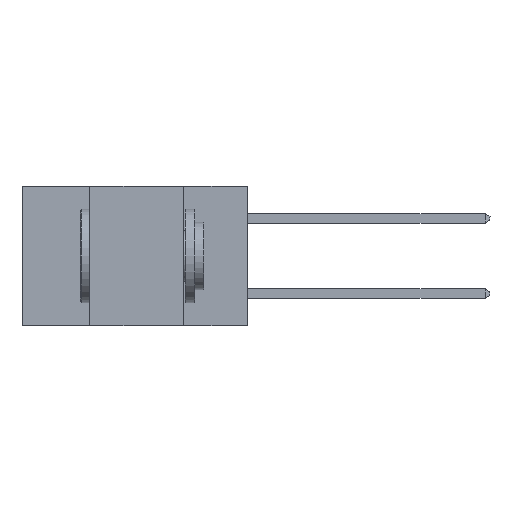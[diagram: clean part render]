
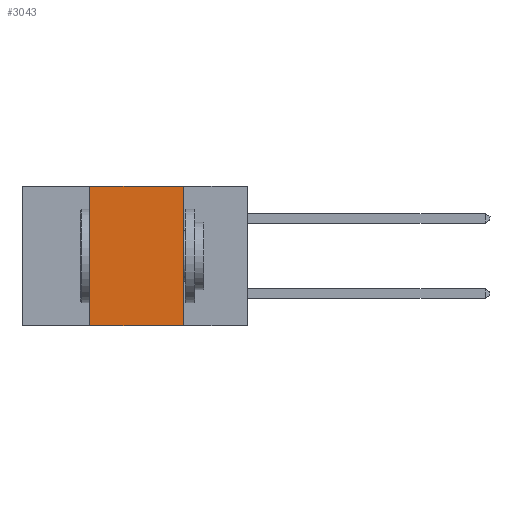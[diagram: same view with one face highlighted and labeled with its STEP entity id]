
A CAD part, left-side view. The second image highlights one B-rep face of the part: STEP entity #3043.
In plain terms, the highlighted planar face has unit normal (-1, 0, 0).
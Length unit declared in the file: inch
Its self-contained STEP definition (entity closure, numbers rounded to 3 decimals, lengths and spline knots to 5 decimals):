
#281 = EDGE_CURVE ( 'NONE', #7087, #9603, #7004, .T. ) ;
#705 = LINE ( 'NONE', #3749, #7884 ) ;
#1080 = PLANE ( 'NONE',  #6649 ) ;
#1147 = EDGE_CURVE ( 'NONE', #7087, #3100, #9301, .T. ) ;
#1456 = VERTEX_POINT ( 'NONE', #3692 ) ;
#1978 = DIRECTION ( 'NONE',  ( 1., 0., 0. ) ) ;
#2467 = DIRECTION ( 'NONE',  ( 0., 0., 1. ) ) ;
#2576 = FACE_OUTER_BOUND ( 'NONE', #8506, .T. ) ;
#3043 = ADVANCED_FACE ( 'NONE', ( #2576 ), #1080, .F. ) ;
#3100 = VERTEX_POINT ( 'NONE', #5658 ) ;
#3257 = LINE ( 'NONE', #4145, #5069 ) ;
#3325 = CARTESIAN_POINT ( 'NONE',  ( 0., 0.42, -0.37 ) ) ;
#3459 = ORIENTED_EDGE ( 'NONE', *, *, #281, .T. ) ;
#3510 = EDGE_CURVE ( 'NONE', #1456, #9603, #3257, .T. ) ;
#3692 = CARTESIAN_POINT ( 'NONE',  ( 0., 0.17, 0. ) ) ;
#3749 = CARTESIAN_POINT ( 'NONE',  ( 0., 0.6, 0. ) ) ;
#4145 = CARTESIAN_POINT ( 'NONE',  ( 0., 0.17, -0.37 ) ) ;
#4190 = DIRECTION ( 'NONE',  ( 0., 0., -1. ) ) ;
#4514 = CARTESIAN_POINT ( 'NONE',  ( 0., 0.17, -0.37 ) ) ;
#5069 = VECTOR ( 'NONE', #4190, 39.37008 ) ;
#5538 = ORIENTED_EDGE ( 'NONE', *, *, #7918, .F. ) ;
#5658 = CARTESIAN_POINT ( 'NONE',  ( 0., 0.42, 0. ) ) ;
#6241 = ORIENTED_EDGE ( 'NONE', *, *, #1147, .F. ) ;
#6649 = AXIS2_PLACEMENT_3D ( 'NONE', #8657, #1978, #8007 ) ;
#7004 = LINE ( 'NONE', #8058, #9038 ) ;
#7087 = VERTEX_POINT ( 'NONE', #3325 ) ;
#7401 = VECTOR ( 'NONE', #2467, 39.37008 ) ;
#7505 = DIRECTION ( 'NONE',  ( 0., -1., 0. ) ) ;
#7859 = CARTESIAN_POINT ( 'NONE',  ( 0., 0.42, -0.37 ) ) ;
#7884 = VECTOR ( 'NONE', #7505, 39.37008 ) ;
#7918 = EDGE_CURVE ( 'NONE', #3100, #1456, #705, .T. ) ;
#8007 = DIRECTION ( 'NONE',  ( 0., 0., -1. ) ) ;
#8058 = CARTESIAN_POINT ( 'NONE',  ( 0., 0.6, -0.37 ) ) ;
#8506 = EDGE_LOOP ( 'NONE', ( #9796, #5538, #6241, #3459 ) ) ;
#8601 = DIRECTION ( 'NONE',  ( 0., -1., 0. ) ) ;
#8657 = CARTESIAN_POINT ( 'NONE',  ( 0., 0.6, 0. ) ) ;
#9038 = VECTOR ( 'NONE', #8601, 39.37008 ) ;
#9301 = LINE ( 'NONE', #7859, #7401 ) ;
#9603 = VERTEX_POINT ( 'NONE', #4514 ) ;
#9796 = ORIENTED_EDGE ( 'NONE', *, *, #3510, .F. ) ;
